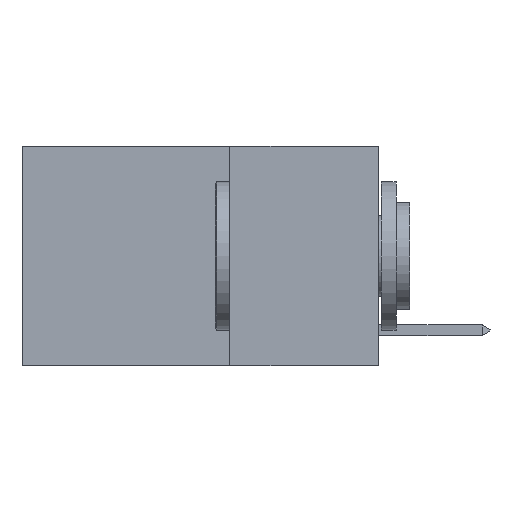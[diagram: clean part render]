
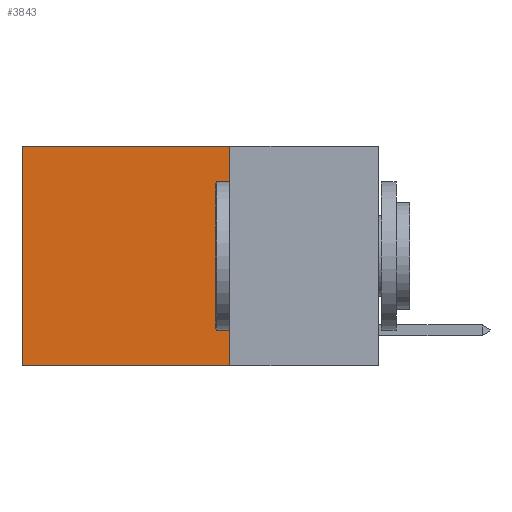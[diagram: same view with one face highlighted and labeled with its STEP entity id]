
A CAD part, left-side view. The second image highlights one B-rep face of the part: STEP entity #3843.
In plain terms, the highlighted planar face has unit normal (-1, 0, 0).
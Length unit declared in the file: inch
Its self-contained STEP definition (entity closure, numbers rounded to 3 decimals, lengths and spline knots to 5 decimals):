
#92 = EDGE_CURVE ( 'NONE', #301, #11856, #4849, .T. ) ;
#301 = VERTEX_POINT ( 'NONE', #8570 ) ;
#502 = DIRECTION ( 'NONE',  ( 0., 0., -1. ) ) ;
#790 = FACE_OUTER_BOUND ( 'NONE', #7753, .T. ) ;
#1676 = CARTESIAN_POINT ( 'NONE',  ( 0.2625, 0.25, 0. ) ) ;
#2225 = VERTEX_POINT ( 'NONE', #12690 ) ;
#2561 = ORIENTED_EDGE ( 'NONE', *, *, #12054, .T. ) ;
#3836 = PLANE ( 'NONE',  #5726 ) ;
#3843 = ADVANCED_FACE ( 'NONE', ( #790 ), #3836, .F. ) ;
#4160 = EDGE_CURVE ( 'NONE', #2225, #301, #8975, .T. ) ;
#4331 = DIRECTION ( 'NONE',  ( 0., 1., 0. ) ) ;
#4849 = LINE ( 'NONE', #12897, #9322 ) ;
#5002 = DIRECTION ( 'NONE',  ( 1., 0., 0. ) ) ;
#5144 = DIRECTION ( 'NONE',  ( 0., 1., 0. ) ) ;
#5620 = DIRECTION ( 'NONE',  ( 0., 0., -1. ) ) ;
#5726 = AXIS2_PLACEMENT_3D ( 'NONE', #1676, #5002, #8037 ) ;
#5914 = LINE ( 'NONE', #10172, #10074 ) ;
#6257 = ORIENTED_EDGE ( 'NONE', *, *, #4160, .F. ) ;
#6451 = LINE ( 'NONE', #8467, #11815 ) ;
#7753 = EDGE_LOOP ( 'NONE', ( #2561, #9772, #6257, #8064 ) ) ;
#8037 = DIRECTION ( 'NONE',  ( 0., 0., -1. ) ) ;
#8064 = ORIENTED_EDGE ( 'NONE', *, *, #9933, .T. ) ;
#8230 = VERTEX_POINT ( 'NONE', #11640 ) ;
#8467 = CARTESIAN_POINT ( 'NONE',  ( 0.2625, 0.25, 0. ) ) ;
#8570 = CARTESIAN_POINT ( 'NONE',  ( 0.2625, 0.25, -0.37 ) ) ;
#8975 = LINE ( 'NONE', #13300, #13106 ) ;
#9322 = VECTOR ( 'NONE', #4331, 39.37008 ) ;
#9772 = ORIENTED_EDGE ( 'NONE', *, *, #92, .F. ) ;
#9933 = EDGE_CURVE ( 'NONE', #2225, #8230, #6451, .T. ) ;
#10074 = VECTOR ( 'NONE', #502, 39.37008 ) ;
#10172 = CARTESIAN_POINT ( 'NONE',  ( 0.2625, 0.6, 0. ) ) ;
#11640 = CARTESIAN_POINT ( 'NONE',  ( 0.2625, 0.6, 0. ) ) ;
#11815 = VECTOR ( 'NONE', #5144, 39.37008 ) ;
#11856 = VERTEX_POINT ( 'NONE', #11967 ) ;
#11967 = CARTESIAN_POINT ( 'NONE',  ( 0.2625, 0.6, -0.37 ) ) ;
#12054 = EDGE_CURVE ( 'NONE', #8230, #11856, #5914, .T. ) ;
#12690 = CARTESIAN_POINT ( 'NONE',  ( 0.2625, 0.25, 0. ) ) ;
#12897 = CARTESIAN_POINT ( 'NONE',  ( 0.2625, 0.25, -0.37 ) ) ;
#13106 = VECTOR ( 'NONE', #5620, 39.37008 ) ;
#13300 = CARTESIAN_POINT ( 'NONE',  ( 0.2625, 0.25, 0. ) ) ;
